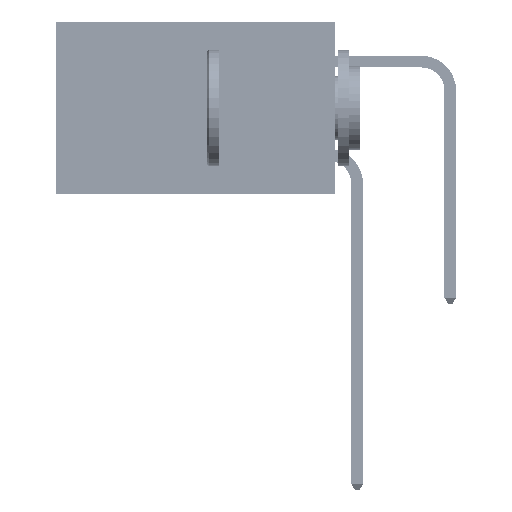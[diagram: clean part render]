
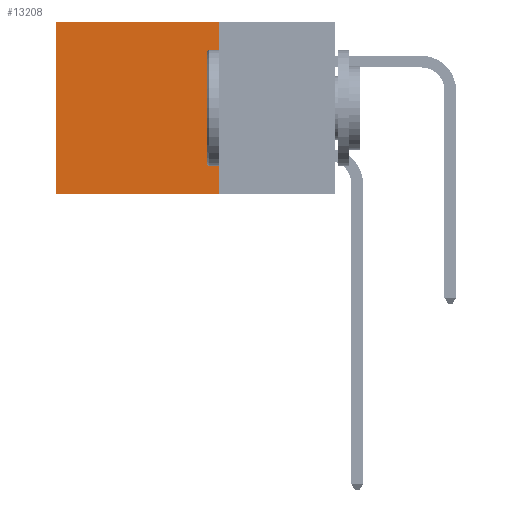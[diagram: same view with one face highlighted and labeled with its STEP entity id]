
A CAD part, left-side view. The second image highlights one B-rep face of the part: STEP entity #13208.
In plain terms, the highlighted planar face has unit normal (-1, 0, 0).
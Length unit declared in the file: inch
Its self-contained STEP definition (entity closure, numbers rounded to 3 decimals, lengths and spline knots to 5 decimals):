
#731 = LINE ( 'NONE', #45362, #20258 ) ;
#2705 = LINE ( 'NONE', #2730, #42804 ) ;
#2730 = CARTESIAN_POINT ( 'NONE',  ( 0.2875, 0.25, -0.37 ) ) ;
#4513 = ORIENTED_EDGE ( 'NONE', *, *, #37993, .T. ) ;
#6208 = ORIENTED_EDGE ( 'NONE', *, *, #29504, .F. ) ;
#6305 = LINE ( 'NONE', #23911, #15426 ) ;
#6757 = ORIENTED_EDGE ( 'NONE', *, *, #7541, .F. ) ;
#7115 = FACE_OUTER_BOUND ( 'NONE', #13913, .T. ) ;
#7541 = EDGE_CURVE ( 'NONE', #40646, #29501, #2705, .T. ) ;
#7571 = DIRECTION ( 'NONE',  ( 0., 1., 0. ) ) ;
#8099 = CARTESIAN_POINT ( 'NONE',  ( 0.2875, 0.25, 0. ) ) ;
#8462 = CARTESIAN_POINT ( 'NONE',  ( 0.2875, 0.6, -0.37 ) ) ;
#8900 = CARTESIAN_POINT ( 'NONE',  ( 0.2875, 0.6, 0. ) ) ;
#10864 = PLANE ( 'NONE',  #35754 ) ;
#11314 = CARTESIAN_POINT ( 'NONE',  ( 0.2875, 0.25, 0. ) ) ;
#13208 = ADVANCED_FACE ( 'NONE', ( #7115 ), #10864, .F. ) ;
#13913 = EDGE_LOOP ( 'NONE', ( #41876, #6757, #6208, #4513 ) ) ;
#14773 = DIRECTION ( 'NONE',  ( 0., 0., -1. ) ) ;
#15426 = VECTOR ( 'NONE', #20166, 39.37008 ) ;
#17871 = LINE ( 'NONE', #11314, #24583 ) ;
#18249 = DIRECTION ( 'NONE',  ( 0., 0., -1. ) ) ;
#20166 = DIRECTION ( 'NONE',  ( 0., 0., -1. ) ) ;
#20258 = VECTOR ( 'NONE', #18249, 39.37008 ) ;
#23911 = CARTESIAN_POINT ( 'NONE',  ( 0.2875, 0.25, 0. ) ) ;
#24583 = VECTOR ( 'NONE', #7571, 39.37008 ) ;
#27745 = CARTESIAN_POINT ( 'NONE',  ( 0.2875, 0.25, -0.37 ) ) ;
#29501 = VERTEX_POINT ( 'NONE', #8462 ) ;
#29504 = EDGE_CURVE ( 'NONE', #40596, #40646, #6305, .T. ) ;
#29883 = EDGE_CURVE ( 'NONE', #42168, #29501, #731, .T. ) ;
#35754 = AXIS2_PLACEMENT_3D ( 'NONE', #45596, #37981, #14773 ) ;
#37981 = DIRECTION ( 'NONE',  ( 1., 0., 0. ) ) ;
#37993 = EDGE_CURVE ( 'NONE', #40596, #42168, #17871, .T. ) ;
#40596 = VERTEX_POINT ( 'NONE', #8099 ) ;
#40646 = VERTEX_POINT ( 'NONE', #27745 ) ;
#41876 = ORIENTED_EDGE ( 'NONE', *, *, #29883, .T. ) ;
#42168 = VERTEX_POINT ( 'NONE', #8900 ) ;
#42804 = VECTOR ( 'NONE', #45501, 39.37008 ) ;
#45362 = CARTESIAN_POINT ( 'NONE',  ( 0.2875, 0.6, 0. ) ) ;
#45501 = DIRECTION ( 'NONE',  ( 0., 1., 0. ) ) ;
#45596 = CARTESIAN_POINT ( 'NONE',  ( 0.2875, 0.25, 0. ) ) ;
